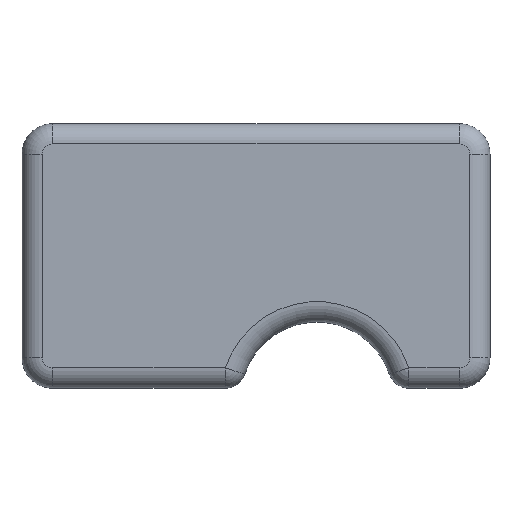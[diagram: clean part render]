
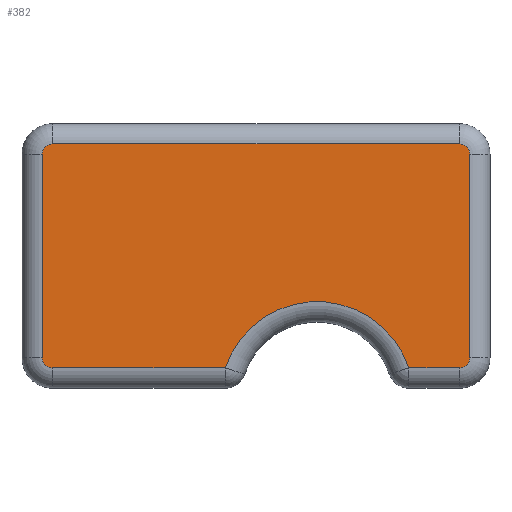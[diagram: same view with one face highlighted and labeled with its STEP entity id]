
A CAD part, top view. The second image highlights one B-rep face of the part: STEP entity #382.
In plain terms, the highlighted planar face has unit normal (0, 0, 1).
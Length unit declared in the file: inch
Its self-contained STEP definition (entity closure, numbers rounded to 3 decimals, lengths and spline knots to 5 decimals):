
#12 = CARTESIAN_POINT ( 'NONE',  ( 0.51181, -0.07874, 0.23031 ) ) ;
#13 = CARTESIAN_POINT ( 'NONE',  ( 0., 0.41339, 0.23031 ) ) ;
#20 = CARTESIAN_POINT ( 'NONE',  ( -0.01969, 0., 0.23031 ) ) ;
#23 = DIRECTION ( 'NONE',  ( 0., 0., 1. ) ) ;
#62 = DIRECTION ( 'NONE',  ( 1., 0., 0. ) ) ;
#67 = DIRECTION ( 'NONE',  ( 0., 0., 1. ) ) ;
#77 = LINE ( 'NONE', #13, #205 ) ;
#90 = AXIS2_PLACEMENT_3D ( 'NONE', #568, #233, #630 ) ;
#91 = VECTOR ( 'NONE', #325, 39.37008 ) ;
#102 = AXIS2_PLACEMENT_3D ( 'NONE', #383, #67, #436 ) ;
#117 = ORIENTED_EDGE ( 'NONE', *, *, #278, .T. ) ;
#118 = AXIS2_PLACEMENT_3D ( 'NONE', #498, #173, #558 ) ;
#125 = AXIS2_PLACEMENT_3D ( 'NONE', #430, #377, #555 ) ;
#130 = VERTEX_POINT ( 'NONE', #462 ) ;
#135 = AXIS2_PLACEMENT_3D ( 'NONE', #336, #23, #393 ) ;
#139 = AXIS2_PLACEMENT_3D ( 'NONE', #12, #381, #62 ) ;
#144 = CARTESIAN_POINT ( 'NONE',  ( 0., -0.01969, 0.23031 ) ) ;
#170 = PLANE ( 'NONE',  #125 ) ;
#173 = DIRECTION ( 'NONE',  ( 0., 0., 1. ) ) ;
#176 = ORIENTED_EDGE ( 'NONE', *, *, #406, .T. ) ;
#177 = ORIENTED_EDGE ( 'NONE', *, *, #370, .T. ) ;
#187 = VERTEX_POINT ( 'NONE', #351 ) ;
#190 = CIRCLE ( 'NONE', #135, 0.01969 ) ;
#205 = VECTOR ( 'NONE', #226, 39.37008 ) ;
#226 = DIRECTION ( 'NONE',  ( -1., 0., 0. ) ) ;
#233 = DIRECTION ( 'NONE',  ( 0., 0., 1. ) ) ;
#240 = LINE ( 'NONE', #551, #91 ) ;
#251 = CARTESIAN_POINT ( 'NONE',  ( -0.01969, 0.3937, 0.23031 ) ) ;
#254 = ORIENTED_EDGE ( 'NONE', *, *, #456, .T. ) ;
#262 = ORIENTED_EDGE ( 'NONE', *, *, #391, .T. ) ;
#269 = VERTEX_POINT ( 'NONE', #251 ) ;
#278 = EDGE_CURVE ( 'NONE', #367, #419, #603, .T. ) ;
#281 = CARTESIAN_POINT ( 'NONE',  ( -0.01969, 0., 0.23031 ) ) ;
#284 = VERTEX_POINT ( 'NONE', #654 ) ;
#293 = VERTEX_POINT ( 'NONE', #302 ) ;
#302 = CARTESIAN_POINT ( 'NONE',  ( 0., 0.41339, 0.23031 ) ) ;
#307 = VECTOR ( 'NONE', #571, 39.37008 ) ;
#319 = EDGE_LOOP ( 'NONE', ( #177, #448, #117, #262, #468, #176, #626, #650, #346, #254 ) ) ;
#325 = DIRECTION ( 'NONE',  ( 1., 0., 0. ) ) ;
#336 = CARTESIAN_POINT ( 'NONE',  ( 0., 0., 0.23031 ) ) ;
#346 = ORIENTED_EDGE ( 'NONE', *, *, #450, .T. ) ;
#351 = CARTESIAN_POINT ( 'NONE',  ( 0.33437, -0.01969, 0.23031 ) ) ;
#367 = VERTEX_POINT ( 'NONE', #708 ) ;
#369 = FACE_OUTER_BOUND ( 'NONE', #319, .T. ) ;
#370 = EDGE_CURVE ( 'NONE', #540, #187, #240, .T. ) ;
#377 = DIRECTION ( 'NONE',  ( 0., 0., 1. ) ) ;
#381 = DIRECTION ( 'NONE',  ( 0., 0., -1. ) ) ;
#382 = ADVANCED_FACE ( 'NONE', ( #369 ), #170, .T. ) ;
#383 = CARTESIAN_POINT ( 'NONE',  ( 0.7874, 0.3937, 0.23031 ) ) ;
#384 = EDGE_CURVE ( 'NONE', #187, #367, #530, .T. ) ;
#390 = CARTESIAN_POINT ( 'NONE',  ( 0.80709, 0., 0.23031 ) ) ;
#391 = EDGE_CURVE ( 'NONE', #419, #440, #666, .T. ) ;
#393 = DIRECTION ( 'NONE',  ( 1., 0., 0. ) ) ;
#401 = EDGE_CURVE ( 'NONE', #440, #284, #655, .T. ) ;
#406 = EDGE_CURVE ( 'NONE', #284, #130, #514, .T. ) ;
#412 = EDGE_CURVE ( 'NONE', #130, #293, #77, .T. ) ;
#419 = VERTEX_POINT ( 'NONE', #502 ) ;
#424 = CARTESIAN_POINT ( 'NONE',  ( 0., -0.01969, 0.23031 ) ) ;
#430 = CARTESIAN_POINT ( 'NONE',  ( 0., 0., 0.23031 ) ) ;
#432 = EDGE_CURVE ( 'NONE', #293, #269, #640, .T. ) ;
#436 = DIRECTION ( 'NONE',  ( 1., 0., 0. ) ) ;
#440 = VERTEX_POINT ( 'NONE', #390 ) ;
#448 = ORIENTED_EDGE ( 'NONE', *, *, #384, .T. ) ;
#450 = EDGE_CURVE ( 'NONE', #269, #707, #455, .T. ) ;
#455 = LINE ( 'NONE', #20, #307 ) ;
#456 = EDGE_CURVE ( 'NONE', #707, #540, #190, .T. ) ;
#462 = CARTESIAN_POINT ( 'NONE',  ( 0.7874, 0.41339, 0.23031 ) ) ;
#468 = ORIENTED_EDGE ( 'NONE', *, *, #401, .T. ) ;
#472 = DIRECTION ( 'NONE',  ( 1., 0., 0. ) ) ;
#490 = VECTOR ( 'NONE', #624, 39.37008 ) ;
#498 = CARTESIAN_POINT ( 'NONE',  ( 0.7874, 0., 0.23031 ) ) ;
#502 = CARTESIAN_POINT ( 'NONE',  ( 0.7874, -0.01969, 0.23031 ) ) ;
#514 = CIRCLE ( 'NONE', #102, 0.01969 ) ;
#530 = CIRCLE ( 'NONE', #139, 0.18701 ) ;
#540 = VERTEX_POINT ( 'NONE', #424 ) ;
#551 = CARTESIAN_POINT ( 'NONE',  ( 0., -0.01969, 0.23031 ) ) ;
#555 = DIRECTION ( 'NONE',  ( 1., 0., 0. ) ) ;
#558 = DIRECTION ( 'NONE',  ( 1., 0., 0. ) ) ;
#568 = CARTESIAN_POINT ( 'NONE',  ( 0., 0.3937, 0.23031 ) ) ;
#571 = DIRECTION ( 'NONE',  ( 0., -1., 0. ) ) ;
#590 = VECTOR ( 'NONE', #472, 39.37008 ) ;
#603 = LINE ( 'NONE', #144, #590 ) ;
#624 = DIRECTION ( 'NONE',  ( 0., 1., 0. ) ) ;
#626 = ORIENTED_EDGE ( 'NONE', *, *, #412, .T. ) ;
#630 = DIRECTION ( 'NONE',  ( 1., 0., 0. ) ) ;
#640 = CIRCLE ( 'NONE', #90, 0.01969 ) ;
#650 = ORIENTED_EDGE ( 'NONE', *, *, #432, .T. ) ;
#654 = CARTESIAN_POINT ( 'NONE',  ( 0.80709, 0.3937, 0.23031 ) ) ;
#655 = LINE ( 'NONE', #673, #490 ) ;
#666 = CIRCLE ( 'NONE', #118, 0.01969 ) ;
#673 = CARTESIAN_POINT ( 'NONE',  ( 0.80709, 0., 0.23031 ) ) ;
#707 = VERTEX_POINT ( 'NONE', #281 ) ;
#708 = CARTESIAN_POINT ( 'NONE',  ( 0.68925, -0.01969, 0.23031 ) ) ;
